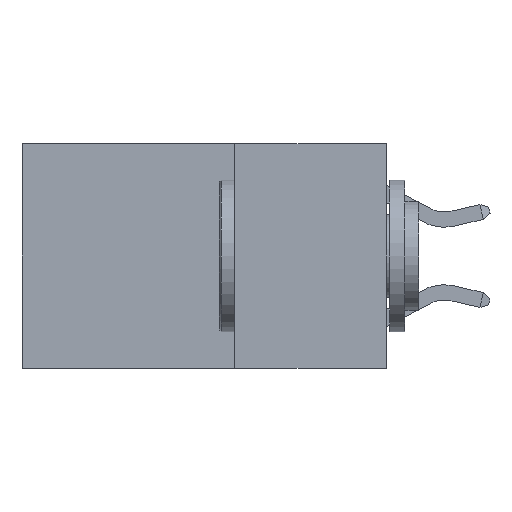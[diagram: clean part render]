
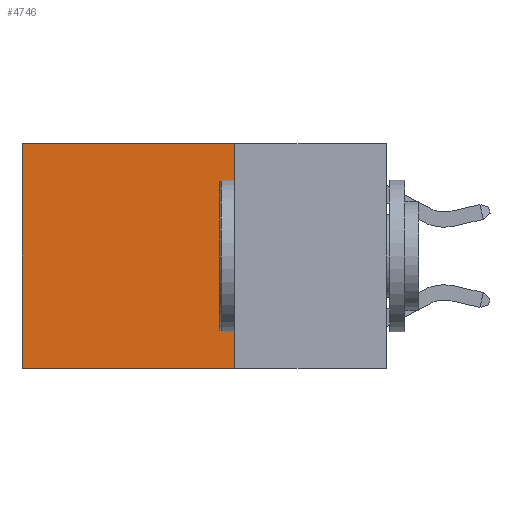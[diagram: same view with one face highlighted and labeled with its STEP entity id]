
A CAD part, left-side view. The second image highlights one B-rep face of the part: STEP entity #4746.
In plain terms, the highlighted planar face has unit normal (-1, 0, 0).
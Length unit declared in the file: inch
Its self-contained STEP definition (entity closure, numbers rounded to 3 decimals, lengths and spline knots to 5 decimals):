
#48 = CARTESIAN_POINT ( 'NONE',  ( 0.2625, 0.25, -0.37 ) ) ;
#248 = VECTOR ( 'NONE', #7793, 39.37008 ) ;
#547 = CARTESIAN_POINT ( 'NONE',  ( 0.2625, 0.25, 0. ) ) ;
#797 = EDGE_LOOP ( 'NONE', ( #3539, #7923, #1530, #6129 ) ) ;
#906 = CARTESIAN_POINT ( 'NONE',  ( 0.2625, 0.25, 0. ) ) ;
#971 = FACE_OUTER_BOUND ( 'NONE', #797, .T. ) ;
#1343 = CARTESIAN_POINT ( 'NONE',  ( 0.2625, 0.25, 0. ) ) ;
#1530 = ORIENTED_EDGE ( 'NONE', *, *, #3568, .F. ) ;
#1587 = VERTEX_POINT ( 'NONE', #48 ) ;
#1857 = LINE ( 'NONE', #6653, #7085 ) ;
#2140 = VERTEX_POINT ( 'NONE', #10265 ) ;
#2307 = EDGE_CURVE ( 'NONE', #3893, #2140, #1857, .T. ) ;
#2694 = CARTESIAN_POINT ( 'NONE',  ( 0.2625, 0.25, 0. ) ) ;
#2741 = LINE ( 'NONE', #2694, #6926 ) ;
#3322 = EDGE_CURVE ( 'NONE', #1587, #2140, #4526, .T. ) ;
#3539 = ORIENTED_EDGE ( 'NONE', *, *, #2307, .T. ) ;
#3568 = EDGE_CURVE ( 'NONE', #4548, #1587, #2741, .T. ) ;
#3841 = DIRECTION ( 'NONE',  ( 0., 1., 0. ) ) ;
#3893 = VERTEX_POINT ( 'NONE', #7928 ) ;
#4174 = DIRECTION ( 'NONE',  ( 1., 0., 0. ) ) ;
#4526 = LINE ( 'NONE', #10310, #248 ) ;
#4548 = VERTEX_POINT ( 'NONE', #1343 ) ;
#4746 = ADVANCED_FACE ( 'NONE', ( #971 ), #5795, .F. ) ;
#5488 = LINE ( 'NONE', #547, #6438 ) ;
#5795 = PLANE ( 'NONE',  #10211 ) ;
#5932 = EDGE_CURVE ( 'NONE', #4548, #3893, #5488, .T. ) ;
#6129 = ORIENTED_EDGE ( 'NONE', *, *, #5932, .T. ) ;
#6438 = VECTOR ( 'NONE', #3841, 39.37008 ) ;
#6653 = CARTESIAN_POINT ( 'NONE',  ( 0.2625, 0.6, 0. ) ) ;
#6926 = VECTOR ( 'NONE', #9271, 39.37008 ) ;
#7085 = VECTOR ( 'NONE', #9931, 39.37008 ) ;
#7446 = DIRECTION ( 'NONE',  ( 0., 0., -1. ) ) ;
#7793 = DIRECTION ( 'NONE',  ( 0., 1., 0. ) ) ;
#7923 = ORIENTED_EDGE ( 'NONE', *, *, #3322, .F. ) ;
#7928 = CARTESIAN_POINT ( 'NONE',  ( 0.2625, 0.6, 0. ) ) ;
#9271 = DIRECTION ( 'NONE',  ( 0., 0., -1. ) ) ;
#9931 = DIRECTION ( 'NONE',  ( 0., 0., -1. ) ) ;
#10211 = AXIS2_PLACEMENT_3D ( 'NONE', #906, #4174, #7446 ) ;
#10265 = CARTESIAN_POINT ( 'NONE',  ( 0.2625, 0.6, -0.37 ) ) ;
#10310 = CARTESIAN_POINT ( 'NONE',  ( 0.2625, 0.25, -0.37 ) ) ;
